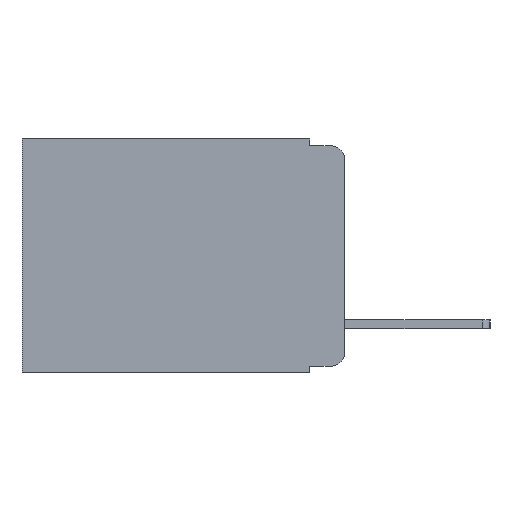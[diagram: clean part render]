
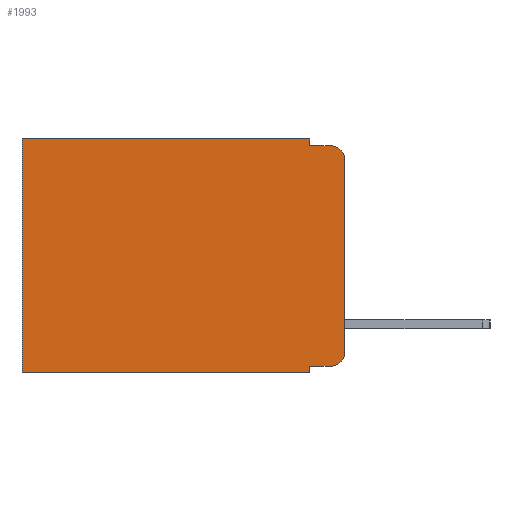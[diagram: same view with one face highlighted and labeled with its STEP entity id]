
A CAD part, left-side view. The second image highlights one B-rep face of the part: STEP entity #1993.
In plain terms, the highlighted planar face has unit normal (-1, 0, 0).
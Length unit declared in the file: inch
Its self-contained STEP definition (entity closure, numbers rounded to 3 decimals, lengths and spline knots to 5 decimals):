
#97 = CARTESIAN_POINT ( 'NONE',  ( 0.298, 0., -0.343 ) ) ;
#414 = EDGE_CURVE ( 'NONE', #6092, #2783, #10792, .T. ) ;
#491 = CARTESIAN_POINT ( 'NONE',  ( 0.298, 0.02, -0.01 ) ) ;
#516 = CARTESIAN_POINT ( 'NONE',  ( 0.298, 0.02, -0.313 ) ) ;
#539 = DIRECTION ( 'NONE',  ( 0., 0., -1. ) ) ;
#636 = EDGE_CURVE ( 'NONE', #7423, #2783, #1879, .T. ) ;
#686 = DIRECTION ( 'NONE',  ( 0., 0., -1. ) ) ;
#745 = DIRECTION ( 'NONE',  ( 0., -1., 0. ) ) ;
#746 = VECTOR ( 'NONE', #1428, 39.37008 ) ;
#896 = LINE ( 'NONE', #7065, #9759 ) ;
#929 = CARTESIAN_POINT ( 'NONE',  ( 0.298, 0.051, -0.343 ) ) ;
#982 = LINE ( 'NONE', #2357, #5407 ) ;
#1146 = EDGE_CURVE ( 'NONE', #3943, #5669, #3682, .T. ) ;
#1428 = DIRECTION ( 'NONE',  ( 0., 1., 0. ) ) ;
#1461 = VECTOR ( 'NONE', #745, 39.37008 ) ;
#1607 = EDGE_CURVE ( 'NONE', #3225, #4845, #896, .T. ) ;
#1708 = ORIENTED_EDGE ( 'NONE', *, *, #7061, .F. ) ;
#1801 = ORIENTED_EDGE ( 'NONE', *, *, #3003, .F. ) ;
#1815 = DIRECTION ( 'NONE',  ( 1., 0., 0. ) ) ;
#1879 = CIRCLE ( 'NONE', #7348, 0.02 ) ;
#1993 = ADVANCED_FACE ( 'NONE', ( #6654 ), #3496, .F. ) ;
#2130 = ORIENTED_EDGE ( 'NONE', *, *, #1607, .T. ) ;
#2155 = ORIENTED_EDGE ( 'NONE', *, *, #1146, .F. ) ;
#2212 = ORIENTED_EDGE ( 'NONE', *, *, #6513, .F. ) ;
#2357 = CARTESIAN_POINT ( 'NONE',  ( 0.298, 0.473, 0. ) ) ;
#2400 = CARTESIAN_POINT ( 'NONE',  ( 0.298, 0., 0. ) ) ;
#2407 = EDGE_CURVE ( 'NONE', #6607, #7423, #4634, .T. ) ;
#2533 = VECTOR ( 'NONE', #10985, 39.37008 ) ;
#2783 = VERTEX_POINT ( 'NONE', #7354 ) ;
#2950 = CARTESIAN_POINT ( 'NONE',  ( 0.298, 0.051, -0.01 ) ) ;
#3003 = EDGE_CURVE ( 'NONE', #6607, #3943, #9991, .T. ) ;
#3225 = VERTEX_POINT ( 'NONE', #4488 ) ;
#3319 = CARTESIAN_POINT ( 'NONE',  ( 0.298, 0.051, 0. ) ) ;
#3496 = PLANE ( 'NONE',  #9295 ) ;
#3682 = LINE ( 'NONE', #97, #746 ) ;
#3835 = VECTOR ( 'NONE', #5538, 39.37008 ) ;
#3852 = DIRECTION ( 'NONE',  ( -1., 0., 0. ) ) ;
#3943 = VERTEX_POINT ( 'NONE', #929 ) ;
#4172 = DIRECTION ( 'NONE',  ( 0., 0., -1. ) ) ;
#4199 = EDGE_CURVE ( 'NONE', #4845, #5669, #982, .T. ) ;
#4488 = CARTESIAN_POINT ( 'NONE',  ( 0.298, 0.051, 0. ) ) ;
#4534 = ORIENTED_EDGE ( 'NONE', *, *, #414, .F. ) ;
#4634 = LINE ( 'NONE', #5177, #2533 ) ;
#4845 = VERTEX_POINT ( 'NONE', #9989 ) ;
#4865 = ORIENTED_EDGE ( 'NONE', *, *, #4199, .T. ) ;
#4948 = ORIENTED_EDGE ( 'NONE', *, *, #636, .T. ) ;
#5177 = CARTESIAN_POINT ( 'NONE',  ( 0.298, 0.051, -0.333 ) ) ;
#5407 = VECTOR ( 'NONE', #7554, 39.37008 ) ;
#5492 = VECTOR ( 'NONE', #686, 39.37008 ) ;
#5538 = DIRECTION ( 'NONE',  ( 0., 0., -1. ) ) ;
#5609 = CARTESIAN_POINT ( 'NONE',  ( 0.298, 0.02, -0.333 ) ) ;
#5621 = VERTEX_POINT ( 'NONE', #2950 ) ;
#5669 = VERTEX_POINT ( 'NONE', #7334 ) ;
#6019 = LINE ( 'NONE', #3319, #5492 ) ;
#6021 = CARTESIAN_POINT ( 'NONE',  ( 0.298, 0.051, -0.01 ) ) ;
#6092 = VERTEX_POINT ( 'NONE', #7136 ) ;
#6096 = DIRECTION ( 'NONE',  ( 0., 1., 0. ) ) ;
#6200 = AXIS2_PLACEMENT_3D ( 'NONE', #8915, #3852, #9746 ) ;
#6513 = EDGE_CURVE ( 'NONE', #3225, #5621, #6019, .T. ) ;
#6607 = VERTEX_POINT ( 'NONE', #6940 ) ;
#6654 = FACE_OUTER_BOUND ( 'NONE', #7769, .T. ) ;
#6703 = DIRECTION ( 'NONE',  ( -1., 0., 0. ) ) ;
#6924 = ORIENTED_EDGE ( 'NONE', *, *, #8730, .T. ) ;
#6940 = CARTESIAN_POINT ( 'NONE',  ( 0.298, 0.051, -0.333 ) ) ;
#6956 = DIRECTION ( 'NONE',  ( 0., 0., -1. ) ) ;
#7061 = EDGE_CURVE ( 'NONE', #5621, #9459, #10538, .T. ) ;
#7065 = CARTESIAN_POINT ( 'NONE',  ( 0.298, 0., 0. ) ) ;
#7136 = CARTESIAN_POINT ( 'NONE',  ( 0.298, 0., -0.03 ) ) ;
#7334 = CARTESIAN_POINT ( 'NONE',  ( 0.298, 0.473, -0.343 ) ) ;
#7348 = AXIS2_PLACEMENT_3D ( 'NONE', #516, #6703, #6956 ) ;
#7354 = CARTESIAN_POINT ( 'NONE',  ( 0.298, 0., -0.313 ) ) ;
#7423 = VERTEX_POINT ( 'NONE', #5609 ) ;
#7554 = DIRECTION ( 'NONE',  ( 0., 0., -1. ) ) ;
#7681 = CIRCLE ( 'NONE', #6200, 0.02 ) ;
#7769 = EDGE_LOOP ( 'NONE', ( #4534, #6924, #1708, #2212, #2130, #4865, #2155, #1801, #8787, #4948 ) ) ;
#7807 = VECTOR ( 'NONE', #4172, 39.37008 ) ;
#8730 = EDGE_CURVE ( 'NONE', #6092, #9459, #7681, .T. ) ;
#8747 = CARTESIAN_POINT ( 'NONE',  ( 0.298, 0., 0. ) ) ;
#8787 = ORIENTED_EDGE ( 'NONE', *, *, #2407, .T. ) ;
#8915 = CARTESIAN_POINT ( 'NONE',  ( 0.298, 0.02, -0.03 ) ) ;
#9295 = AXIS2_PLACEMENT_3D ( 'NONE', #8747, #1815, #539 ) ;
#9459 = VERTEX_POINT ( 'NONE', #491 ) ;
#9746 = DIRECTION ( 'NONE',  ( 0., 0., -1. ) ) ;
#9759 = VECTOR ( 'NONE', #6096, 39.37008 ) ;
#9989 = CARTESIAN_POINT ( 'NONE',  ( 0.298, 0.473, 0. ) ) ;
#9991 = LINE ( 'NONE', #10862, #7807 ) ;
#10538 = LINE ( 'NONE', #6021, #1461 ) ;
#10792 = LINE ( 'NONE', #2400, #3835 ) ;
#10862 = CARTESIAN_POINT ( 'NONE',  ( 0.298, 0.051, 0. ) ) ;
#10985 = DIRECTION ( 'NONE',  ( 0., -1., 0. ) ) ;
